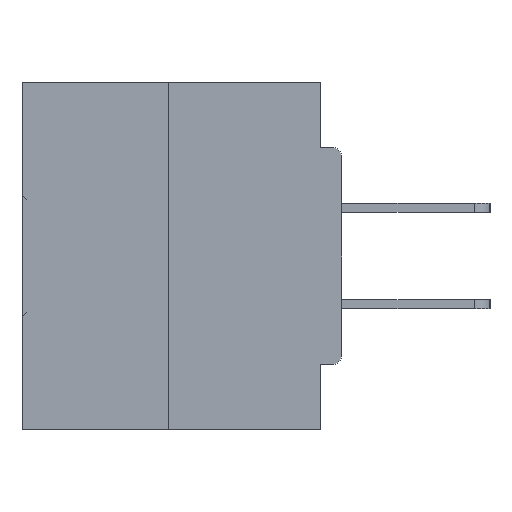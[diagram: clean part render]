
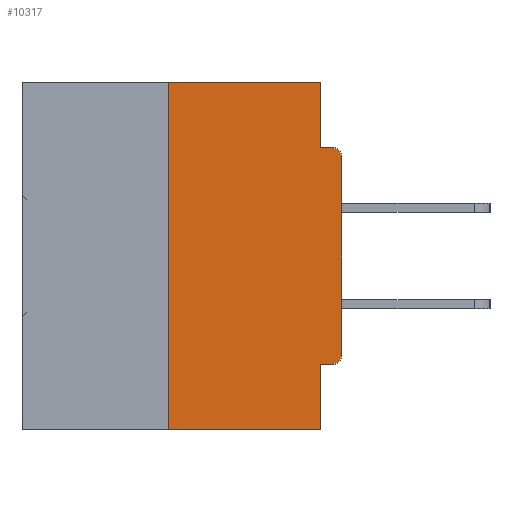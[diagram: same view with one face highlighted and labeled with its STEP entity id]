
A CAD part, left-side view. The second image highlights one B-rep face of the part: STEP entity #10317.
In plain terms, the highlighted planar face has unit normal (-1, 0, 0).
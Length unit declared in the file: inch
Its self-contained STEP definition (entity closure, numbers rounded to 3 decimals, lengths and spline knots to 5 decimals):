
#726 = VECTOR ( 'NONE', #17610, 39.37008 ) ;
#921 = VERTEX_POINT ( 'NONE', #40013 ) ;
#1355 = CARTESIAN_POINT ( 'NONE',  ( 0., 0.031, 0. ) ) ;
#2229 = VECTOR ( 'NONE', #7585, 39.37008 ) ;
#2996 = DIRECTION ( 'NONE',  ( 0., 0., 1. ) ) ;
#3795 = CARTESIAN_POINT ( 'NONE',  ( 0., 0.25, 0. ) ) ;
#4079 = CARTESIAN_POINT ( 'NONE',  ( 0., 0., -0.1085 ) ) ;
#4681 = LINE ( 'NONE', #9990, #726 ) ;
#5969 = CARTESIAN_POINT ( 'NONE',  ( 0., 0., -0.3915 ) ) ;
#6290 = PLANE ( 'NONE',  #28971 ) ;
#7096 = EDGE_LOOP ( 'NONE', ( #8484, #43726, #29730, #39061, #12131, #20722, #36476, #35191, #42274, #32948 ) ) ;
#7585 = DIRECTION ( 'NONE',  ( 0., 0., 1. ) ) ;
#7820 = CARTESIAN_POINT ( 'NONE',  ( 0., 0., -0.4065 ) ) ;
#8340 = DIRECTION ( 'NONE',  ( 0., -1., 0. ) ) ;
#8363 = CARTESIAN_POINT ( 'NONE',  ( 0., 0.031, -0.5 ) ) ;
#8484 = ORIENTED_EDGE ( 'NONE', *, *, #38572, .F. ) ;
#8608 = VECTOR ( 'NONE', #25826, 39.37008 ) ;
#9910 = CARTESIAN_POINT ( 'NONE',  ( 0., 0.015, -0.3915 ) ) ;
#9946 = DIRECTION ( 'NONE',  ( 0., 0., -1. ) ) ;
#9948 = CIRCLE ( 'NONE', #19542, 0.015 ) ;
#9990 = CARTESIAN_POINT ( 'NONE',  ( 0., 0., -0.0935 ) ) ;
#10317 = ADVANCED_FACE ( 'NONE', ( #21743 ), #6290, .F. ) ;
#10534 = CARTESIAN_POINT ( 'NONE',  ( 0., 0.015, -0.0935 ) ) ;
#10877 = LINE ( 'NONE', #43403, #8608 ) ;
#11582 = DIRECTION ( 'NONE',  ( -1., 0., 0. ) ) ;
#12131 = ORIENTED_EDGE ( 'NONE', *, *, #16175, .F. ) ;
#12402 = DIRECTION ( 'NONE',  ( 0., 0., -1. ) ) ;
#13826 = DIRECTION ( 'NONE',  ( -1., 0., 0. ) ) ;
#15595 = VERTEX_POINT ( 'NONE', #17967 ) ;
#16047 = VECTOR ( 'NONE', #40691, 39.37008 ) ;
#16175 = EDGE_CURVE ( 'NONE', #40073, #921, #35196, .T. ) ;
#17610 = DIRECTION ( 'NONE',  ( 0., -1., 0. ) ) ;
#17967 = CARTESIAN_POINT ( 'NONE',  ( 0., 0.25, 0. ) ) ;
#18289 = CARTESIAN_POINT ( 'NONE',  ( 0., 0.015, -0.1085 ) ) ;
#19081 = VERTEX_POINT ( 'NONE', #27495 ) ;
#19542 = AXIS2_PLACEMENT_3D ( 'NONE', #18289, #11582, #22227 ) ;
#20722 = ORIENTED_EDGE ( 'NONE', *, *, #34260, .T. ) ;
#20740 = DIRECTION ( 'NONE',  ( 1., 0., 0. ) ) ;
#21743 = FACE_OUTER_BOUND ( 'NONE', #7096, .T. ) ;
#22227 = DIRECTION ( 'NONE',  ( 0., 0., -1. ) ) ;
#23006 = LINE ( 'NONE', #31456, #31424 ) ;
#23344 = VERTEX_POINT ( 'NONE', #37897 ) ;
#23620 = VERTEX_POINT ( 'NONE', #23996 ) ;
#23996 = CARTESIAN_POINT ( 'NONE',  ( 0., 0.031, -0.0935 ) ) ;
#24040 = CARTESIAN_POINT ( 'NONE',  ( 0., 0.031, 0. ) ) ;
#24262 = CIRCLE ( 'NONE', #35702, 0.015 ) ;
#25597 = LINE ( 'NONE', #8363, #16047 ) ;
#25735 = DIRECTION ( 'NONE',  ( 0., 1., 0. ) ) ;
#25826 = DIRECTION ( 'NONE',  ( 0., -1., 0. ) ) ;
#26137 = VERTEX_POINT ( 'NONE', #5969 ) ;
#27495 = CARTESIAN_POINT ( 'NONE',  ( 0., 0.031, -0.5 ) ) ;
#27793 = DIRECTION ( 'NONE',  ( 0., 0., -1. ) ) ;
#27909 = VERTEX_POINT ( 'NONE', #24040 ) ;
#28971 = AXIS2_PLACEMENT_3D ( 'NONE', #45572, #20740, #9946 ) ;
#29730 = ORIENTED_EDGE ( 'NONE', *, *, #33319, .T. ) ;
#30379 = LINE ( 'NONE', #3795, #2229 ) ;
#30590 = EDGE_CURVE ( 'NONE', #23620, #41595, #4681, .T. ) ;
#31424 = VECTOR ( 'NONE', #2996, 39.37008 ) ;
#31456 = CARTESIAN_POINT ( 'NONE',  ( 0., 0., 0. ) ) ;
#32063 = VECTOR ( 'NONE', #12402, 39.37008 ) ;
#32170 = EDGE_CURVE ( 'NONE', #921, #19081, #25597, .T. ) ;
#32932 = LINE ( 'NONE', #33566, #38596 ) ;
#32948 = ORIENTED_EDGE ( 'NONE', *, *, #41919, .F. ) ;
#33319 = EDGE_CURVE ( 'NONE', #23344, #19081, #10877, .T. ) ;
#33566 = CARTESIAN_POINT ( 'NONE',  ( 0., 0.46, 0. ) ) ;
#33700 = LINE ( 'NONE', #1355, #32063 ) ;
#34260 = EDGE_CURVE ( 'NONE', #40073, #26137, #24262, .T. ) ;
#34533 = CARTESIAN_POINT ( 'NONE',  ( 0., 0.015, -0.4065 ) ) ;
#35191 = ORIENTED_EDGE ( 'NONE', *, *, #44896, .T. ) ;
#35196 = LINE ( 'NONE', #7820, #42547 ) ;
#35702 = AXIS2_PLACEMENT_3D ( 'NONE', #9910, #13826, #27793 ) ;
#35725 = EDGE_CURVE ( 'NONE', #26137, #35853, #23006, .T. ) ;
#35853 = VERTEX_POINT ( 'NONE', #4079 ) ;
#36476 = ORIENTED_EDGE ( 'NONE', *, *, #35725, .T. ) ;
#37897 = CARTESIAN_POINT ( 'NONE',  ( 0., 0.25, -0.5 ) ) ;
#38572 = EDGE_CURVE ( 'NONE', #15595, #27909, #32932, .T. ) ;
#38596 = VECTOR ( 'NONE', #8340, 39.37008 ) ;
#39061 = ORIENTED_EDGE ( 'NONE', *, *, #32170, .F. ) ;
#40013 = CARTESIAN_POINT ( 'NONE',  ( 0., 0.031, -0.4065 ) ) ;
#40073 = VERTEX_POINT ( 'NONE', #34533 ) ;
#40691 = DIRECTION ( 'NONE',  ( 0., 0., -1. ) ) ;
#41595 = VERTEX_POINT ( 'NONE', #10534 ) ;
#41919 = EDGE_CURVE ( 'NONE', #27909, #23620, #33700, .T. ) ;
#42274 = ORIENTED_EDGE ( 'NONE', *, *, #30590, .F. ) ;
#42547 = VECTOR ( 'NONE', #25735, 39.37008 ) ;
#42840 = EDGE_CURVE ( 'NONE', #23344, #15595, #30379, .T. ) ;
#43403 = CARTESIAN_POINT ( 'NONE',  ( 0., 0.46, -0.5 ) ) ;
#43726 = ORIENTED_EDGE ( 'NONE', *, *, #42840, .F. ) ;
#44896 = EDGE_CURVE ( 'NONE', #35853, #41595, #9948, .T. ) ;
#45572 = CARTESIAN_POINT ( 'NONE',  ( 0., 0.46, 0. ) ) ;
